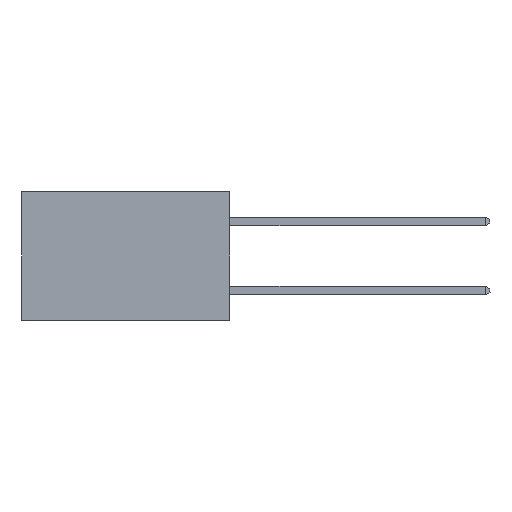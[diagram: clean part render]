
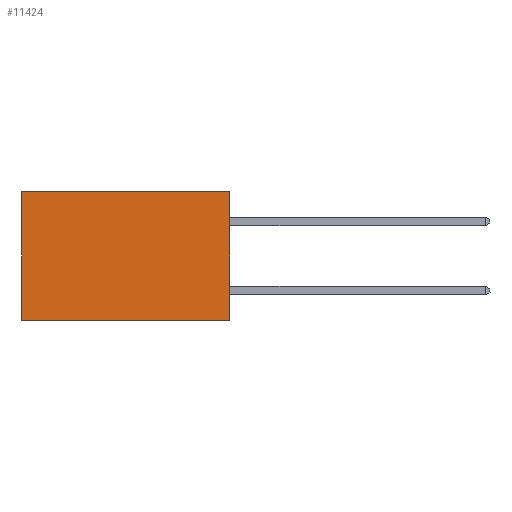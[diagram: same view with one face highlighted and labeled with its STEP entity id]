
A CAD part, left-side view. The second image highlights one B-rep face of the part: STEP entity #11424.
In plain terms, the highlighted planar face has unit normal (-1, 0, 0).
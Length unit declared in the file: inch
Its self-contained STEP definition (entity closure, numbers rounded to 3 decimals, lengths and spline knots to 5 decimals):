
#219 = EDGE_CURVE ( 'NONE', #17200, #13376, #4461, .T. ) ;
#469 = CARTESIAN_POINT ( 'NONE',  ( 0.298, 0.6, 0. ) ) ;
#499 = VECTOR ( 'NONE', #5826, 39.37008 ) ;
#2169 = DIRECTION ( 'NONE',  ( 0., 0., -1. ) ) ;
#2506 = CARTESIAN_POINT ( 'NONE',  ( 0.298, 0., 0. ) ) ;
#2593 = LINE ( 'NONE', #6378, #20191 ) ;
#4461 = LINE ( 'NONE', #2506, #499 ) ;
#4826 = DIRECTION ( 'NONE',  ( 0., 0., -1. ) ) ;
#5248 = LINE ( 'NONE', #20941, #12552 ) ;
#5614 = CARTESIAN_POINT ( 'NONE',  ( 0.298, 0., -0.37 ) ) ;
#5826 = DIRECTION ( 'NONE',  ( 0., 1., 0. ) ) ;
#6378 = CARTESIAN_POINT ( 'NONE',  ( 0.298, 0., 0. ) ) ;
#6608 = PLANE ( 'NONE',  #13044 ) ;
#6665 = EDGE_CURVE ( 'NONE', #21775, #13389, #5248, .T. ) ;
#6858 = CARTESIAN_POINT ( 'NONE',  ( 0.298, 0., 0. ) ) ;
#8212 = DIRECTION ( 'NONE',  ( 0., 0., -1. ) ) ;
#11424 = ADVANCED_FACE ( 'NONE', ( #13459 ), #6608, .F. ) ;
#11564 = ORIENTED_EDGE ( 'NONE', *, *, #6665, .F. ) ;
#11705 = CARTESIAN_POINT ( 'NONE',  ( 0.298, 0., 0. ) ) ;
#12552 = VECTOR ( 'NONE', #14408, 39.37008 ) ;
#12799 = CARTESIAN_POINT ( 'NONE',  ( 0.298, 0.6, -0.37 ) ) ;
#13044 = AXIS2_PLACEMENT_3D ( 'NONE', #11705, #19954, #8212 ) ;
#13376 = VERTEX_POINT ( 'NONE', #15709 ) ;
#13389 = VERTEX_POINT ( 'NONE', #12799 ) ;
#13459 = FACE_OUTER_BOUND ( 'NONE', #17304, .T. ) ;
#14278 = EDGE_CURVE ( 'NONE', #17200, #21775, #2593, .T. ) ;
#14408 = DIRECTION ( 'NONE',  ( 0., 1., 0. ) ) ;
#15709 = CARTESIAN_POINT ( 'NONE',  ( 0.298, 0.6, 0. ) ) ;
#17200 = VERTEX_POINT ( 'NONE', #6858 ) ;
#17304 = EDGE_LOOP ( 'NONE', ( #18648, #11564, #20453, #17475 ) ) ;
#17475 = ORIENTED_EDGE ( 'NONE', *, *, #219, .T. ) ;
#18191 = VECTOR ( 'NONE', #2169, 39.37008 ) ;
#18285 = EDGE_CURVE ( 'NONE', #13376, #13389, #18995, .T. ) ;
#18648 = ORIENTED_EDGE ( 'NONE', *, *, #18285, .T. ) ;
#18995 = LINE ( 'NONE', #469, #18191 ) ;
#19954 = DIRECTION ( 'NONE',  ( 1., 0., 0. ) ) ;
#20191 = VECTOR ( 'NONE', #4826, 39.37008 ) ;
#20453 = ORIENTED_EDGE ( 'NONE', *, *, #14278, .F. ) ;
#20941 = CARTESIAN_POINT ( 'NONE',  ( 0.298, 0., -0.37 ) ) ;
#21775 = VERTEX_POINT ( 'NONE', #5614 ) ;
